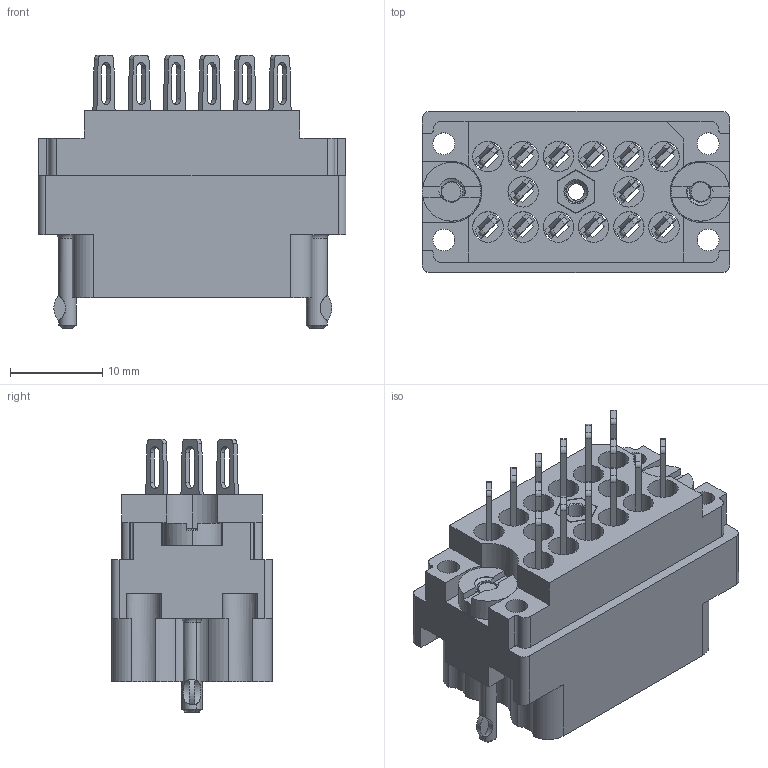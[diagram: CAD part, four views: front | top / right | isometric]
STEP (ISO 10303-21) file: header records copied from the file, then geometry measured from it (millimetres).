
FILE_DESCRIPTION (( 'STEP AP203' ), '1' );
FILE_NAME ('519-014-500-302.STEP', '2020-03-11T15:52:32', ( '' ), ( '' ), 'SwSTEP 2.0', 'SolidWorks 2016', '' );
FILE_SCHEMA (( 'CONFIG_CONTROL_DESIGN' ));
Length unit declared in the file: inch
Products named in the file (7): 516-252-021-102_014; 519-014-500-302; 516-222-020-102_014; 519 Plug Insulator_014; 516-222-020-102_015; 516-252-025-100_516-252-025-100; 516-292-001_500 Contact
Assembly tree (20 placements, depth 2):
  519-014-500-302
    519 Plug Insulator_014
    516-292-001_500 Contact  x14
    516-252-025-100_516-252-025-100
    516-252-021-102_014  x2
    516-222-020-102_014
    516-222-020-102_015
Bounding box: 33.32 x 17.42 x 29.59 mm (x, y, z)
Volume: 5906.7 mm3; surface area: 9599.7 mm2
Topology: 20 solids, 20 shells, 1804 faces, 5159 edges, 3410 vertices
Faces by surface type: plane 984, cylinder 644, bspline 123, cone 49, torus 4
Entity records: 33550 total; most frequent: CARTESIAN_POINT 12209, ORIENTED_EDGE 4418, DIRECTION 4073, EDGE_CURVE 2209, VERTEX_POINT 1452, AXIS2_PLACEMENT_3D 1362, LINE 1349, VECTOR 1349
